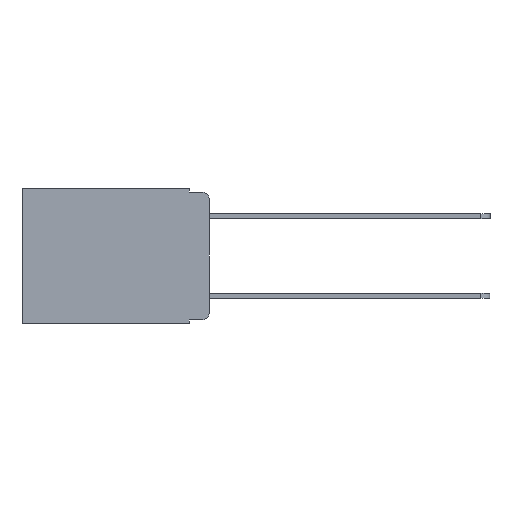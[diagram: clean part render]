
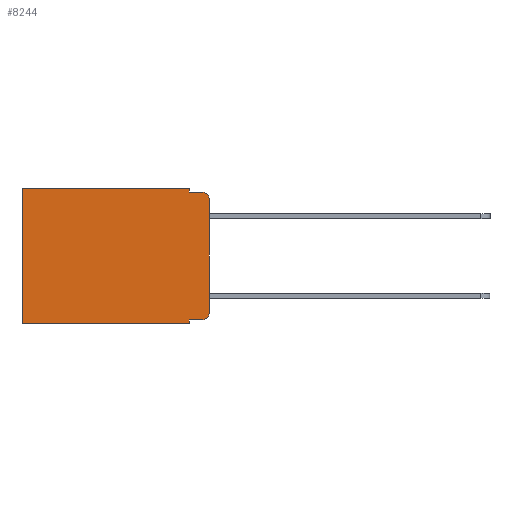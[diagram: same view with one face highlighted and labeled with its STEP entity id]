
A CAD part, left-side view. The second image highlights one B-rep face of the part: STEP entity #8244.
In plain terms, the highlighted planar face has unit normal (-1, 0, 0).
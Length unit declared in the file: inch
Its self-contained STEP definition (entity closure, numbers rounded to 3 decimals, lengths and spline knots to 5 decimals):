
#293 = DIRECTION ( 'NONE',  ( 0., -1., 0. ) ) ;
#548 = CIRCLE ( 'NONE', #4212, 0.02 ) ;
#556 = VERTEX_POINT ( 'NONE', #3706 ) ;
#767 = ORIENTED_EDGE ( 'NONE', *, *, #4104, .T. ) ;
#998 = VERTEX_POINT ( 'NONE', #1852 ) ;
#1010 = VECTOR ( 'NONE', #293, 39.37008 ) ;
#1029 = ORIENTED_EDGE ( 'NONE', *, *, #6072, .T. ) ;
#1191 = CARTESIAN_POINT ( 'NONE',  ( 0.298, 0.473, 0. ) ) ;
#1252 = ORIENTED_EDGE ( 'NONE', *, *, #5349, .F. ) ;
#1406 = ORIENTED_EDGE ( 'NONE', *, *, #9255, .F. ) ;
#1420 = CARTESIAN_POINT ( 'NONE',  ( 0.298, 0., 0. ) ) ;
#1436 = DIRECTION ( 'NONE',  ( -1., 0., 0. ) ) ;
#1452 = CARTESIAN_POINT ( 'NONE',  ( 0.298, 0.02, -0.03 ) ) ;
#1462 = DIRECTION ( 'NONE',  ( 0., 0., -1. ) ) ;
#1468 = VERTEX_POINT ( 'NONE', #1191 ) ;
#1852 = CARTESIAN_POINT ( 'NONE',  ( 0.298, 0.051, -0.343 ) ) ;
#2005 = ORIENTED_EDGE ( 'NONE', *, *, #5939, .F. ) ;
#2011 = CARTESIAN_POINT ( 'NONE',  ( 0.298, 0., 0. ) ) ;
#2306 = DIRECTION ( 'NONE',  ( 0., 0., -1. ) ) ;
#2409 = CIRCLE ( 'NONE', #3777, 0.02 ) ;
#2417 = CARTESIAN_POINT ( 'NONE',  ( 0.298, 0.051, -0.01 ) ) ;
#2518 = DIRECTION ( 'NONE',  ( 0., 1., 0. ) ) ;
#2676 = CARTESIAN_POINT ( 'NONE',  ( 0.298, 0., -0.343 ) ) ;
#2758 = ORIENTED_EDGE ( 'NONE', *, *, #8900, .T. ) ;
#3097 = CARTESIAN_POINT ( 'NONE',  ( 0.298, 0.473, -0.343 ) ) ;
#3151 = CARTESIAN_POINT ( 'NONE',  ( 0.298, 0.051, -0.01 ) ) ;
#3246 = CARTESIAN_POINT ( 'NONE',  ( 0.298, 0., 0. ) ) ;
#3392 = LINE ( 'NONE', #2676, #7100 ) ;
#3407 = DIRECTION ( 'NONE',  ( 0., 1., 0. ) ) ;
#3706 = CARTESIAN_POINT ( 'NONE',  ( 0.298, 0.02, -0.01 ) ) ;
#3728 = VERTEX_POINT ( 'NONE', #3868 ) ;
#3777 = AXIS2_PLACEMENT_3D ( 'NONE', #1452, #1436, #4382 ) ;
#3786 = VECTOR ( 'NONE', #3910, 39.37008 ) ;
#3813 = AXIS2_PLACEMENT_3D ( 'NONE', #1420, #6782, #2306 ) ;
#3868 = CARTESIAN_POINT ( 'NONE',  ( 0.298, 0., -0.03 ) ) ;
#3910 = DIRECTION ( 'NONE',  ( 0., -1., 0. ) ) ;
#3923 = VERTEX_POINT ( 'NONE', #9811 ) ;
#3969 = VECTOR ( 'NONE', #1462, 39.37008 ) ;
#4060 = CARTESIAN_POINT ( 'NONE',  ( 0.298, 0.051, 0. ) ) ;
#4104 = EDGE_CURVE ( 'NONE', #3728, #556, #2409, .T. ) ;
#4185 = VECTOR ( 'NONE', #8874, 39.37008 ) ;
#4194 = LINE ( 'NONE', #4060, #3969 ) ;
#4212 = AXIS2_PLACEMENT_3D ( 'NONE', #6105, #6093, #6073 ) ;
#4382 = DIRECTION ( 'NONE',  ( 0., 0., -1. ) ) ;
#4472 = ORIENTED_EDGE ( 'NONE', *, *, #6053, .T. ) ;
#4535 = LINE ( 'NONE', #6363, #7714 ) ;
#4789 = EDGE_LOOP ( 'NONE', ( #1406, #767, #1252, #2005, #5967, #1029, #5222, #7805, #2758, #4472 ) ) ;
#4906 = CARTESIAN_POINT ( 'NONE',  ( 0.298, 0.051, -0.333 ) ) ;
#5206 = DIRECTION ( 'NONE',  ( 0., 0., -1. ) ) ;
#5222 = ORIENTED_EDGE ( 'NONE', *, *, #9140, .F. ) ;
#5349 = EDGE_CURVE ( 'NONE', #6644, #556, #8629, .T. ) ;
#5716 = EDGE_CURVE ( 'NONE', #9880, #998, #4194, .T. ) ;
#5837 = VERTEX_POINT ( 'NONE', #7503 ) ;
#5939 = EDGE_CURVE ( 'NONE', #3923, #6644, #4535, .T. ) ;
#5967 = ORIENTED_EDGE ( 'NONE', *, *, #7597, .T. ) ;
#6044 = PLANE ( 'NONE',  #3813 ) ;
#6053 = EDGE_CURVE ( 'NONE', #5837, #8317, #548, .T. ) ;
#6072 = EDGE_CURVE ( 'NONE', #1468, #7514, #7823, .T. ) ;
#6073 = DIRECTION ( 'NONE',  ( 0., 0., -1. ) ) ;
#6081 = CARTESIAN_POINT ( 'NONE',  ( 0.298, 0., -0.313 ) ) ;
#6093 = DIRECTION ( 'NONE',  ( -1., 0., 0. ) ) ;
#6105 = CARTESIAN_POINT ( 'NONE',  ( 0.298, 0.02, -0.313 ) ) ;
#6198 = LINE ( 'NONE', #3246, #9722 ) ;
#6363 = CARTESIAN_POINT ( 'NONE',  ( 0.298, 0.051, 0. ) ) ;
#6644 = VERTEX_POINT ( 'NONE', #3151 ) ;
#6782 = DIRECTION ( 'NONE',  ( 1., 0., 0. ) ) ;
#7100 = VECTOR ( 'NONE', #3407, 39.37008 ) ;
#7503 = CARTESIAN_POINT ( 'NONE',  ( 0.298, 0.02, -0.333 ) ) ;
#7514 = VERTEX_POINT ( 'NONE', #3097 ) ;
#7597 = EDGE_CURVE ( 'NONE', #3923, #1468, #6198, .T. ) ;
#7661 = LINE ( 'NONE', #8266, #3786 ) ;
#7714 = VECTOR ( 'NONE', #5206, 39.37008 ) ;
#7805 = ORIENTED_EDGE ( 'NONE', *, *, #5716, .F. ) ;
#7823 = LINE ( 'NONE', #8790, #4185 ) ;
#7879 = LINE ( 'NONE', #2011, #9485 ) ;
#7972 = DIRECTION ( 'NONE',  ( 0., 0., -1. ) ) ;
#8123 = FACE_OUTER_BOUND ( 'NONE', #4789, .T. ) ;
#8244 = ADVANCED_FACE ( 'NONE', ( #8123 ), #6044, .F. ) ;
#8266 = CARTESIAN_POINT ( 'NONE',  ( 0.298, 0.051, -0.333 ) ) ;
#8317 = VERTEX_POINT ( 'NONE', #6081 ) ;
#8629 = LINE ( 'NONE', #2417, #1010 ) ;
#8790 = CARTESIAN_POINT ( 'NONE',  ( 0.298, 0.473, 0. ) ) ;
#8874 = DIRECTION ( 'NONE',  ( 0., 0., -1. ) ) ;
#8900 = EDGE_CURVE ( 'NONE', #9880, #5837, #7661, .T. ) ;
#9140 = EDGE_CURVE ( 'NONE', #998, #7514, #3392, .T. ) ;
#9255 = EDGE_CURVE ( 'NONE', #3728, #8317, #7879, .T. ) ;
#9485 = VECTOR ( 'NONE', #7972, 39.37008 ) ;
#9722 = VECTOR ( 'NONE', #2518, 39.37008 ) ;
#9811 = CARTESIAN_POINT ( 'NONE',  ( 0.298, 0.051, 0. ) ) ;
#9880 = VERTEX_POINT ( 'NONE', #4906 ) ;
